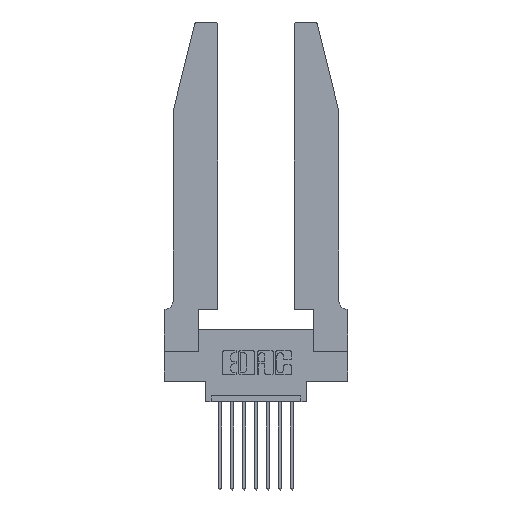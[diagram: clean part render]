
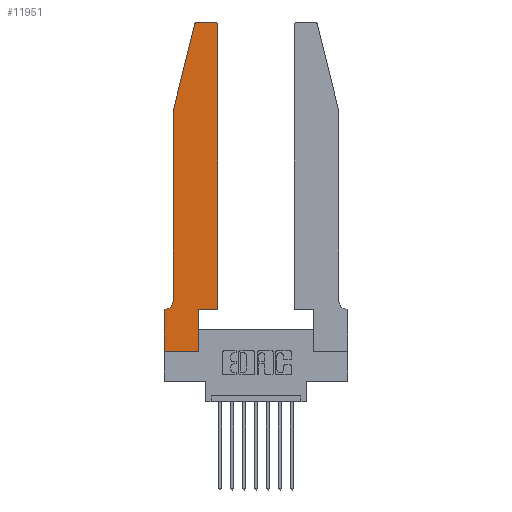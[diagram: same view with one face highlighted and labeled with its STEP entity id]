
A CAD part, top view. The second image highlights one B-rep face of the part: STEP entity #11951.
In plain terms, the highlighted planar face has unit normal (0, 0, 1).
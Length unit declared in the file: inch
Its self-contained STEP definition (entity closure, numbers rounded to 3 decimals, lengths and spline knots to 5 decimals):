
#201 = ORIENTED_EDGE ( 'NONE', *, *, #12708, .T. ) ;
#231 = CARTESIAN_POINT ( 'NONE',  ( 0.2865, 0.35, 0.37 ) ) ;
#441 = VECTOR ( 'NONE', #7008, 39.37008 ) ;
#580 = VECTOR ( 'NONE', #14344, 39.37008 ) ;
#858 = EDGE_CURVE ( 'NONE', #9339, #12194, #10511, .T. ) ;
#965 = EDGE_CURVE ( 'NONE', #3854, #10141, #13375, .T. ) ;
#1080 = CARTESIAN_POINT ( 'NONE',  ( 0.0755, 2., 0.37 ) ) ;
#1188 = FACE_OUTER_BOUND ( 'NONE', #7702, .T. ) ;
#1193 = DIRECTION ( 'NONE',  ( 0., -1., 0. ) ) ;
#1369 = CARTESIAN_POINT ( 'NONE',  ( 0., 0.35, 0.37 ) ) ;
#1457 = VERTEX_POINT ( 'NONE', #10189 ) ;
#1799 = ORIENTED_EDGE ( 'NONE', *, *, #965, .T. ) ;
#1825 = ORIENTED_EDGE ( 'NONE', *, *, #12223, .T. ) ;
#1881 = VECTOR ( 'NONE', #5202, 39.37008 ) ;
#2088 = CIRCLE ( 'NONE', #11531, 0.07 ) ;
#2167 = ORIENTED_EDGE ( 'NONE', *, *, #7016, .T. ) ;
#2403 = EDGE_CURVE ( 'NONE', #10127, #9339, #9746, .T. ) ;
#2482 = CARTESIAN_POINT ( 'NONE',  ( 0., 0., 0.37 ) ) ;
#2566 = LINE ( 'NONE', #8594, #6352 ) ;
#2736 = ORIENTED_EDGE ( 'NONE', *, *, #8646, .T. ) ;
#2794 = LINE ( 'NONE', #10407, #14669 ) ;
#2820 = CARTESIAN_POINT ( 'NONE',  ( 0., 0., 0.37 ) ) ;
#2854 = DIRECTION ( 'NONE',  ( 0., 0., 1. ) ) ;
#2910 = CARTESIAN_POINT ( 'NONE',  ( 0.2865, 0.35, 0.37 ) ) ;
#3718 = ORIENTED_EDGE ( 'NONE', *, *, #12362, .T. ) ;
#3731 = VERTEX_POINT ( 'NONE', #9314 ) ;
#3753 = CARTESIAN_POINT ( 'NONE',  ( 0.0055, 0.35, 0.37 ) ) ;
#3854 = VERTEX_POINT ( 'NONE', #10571 ) ;
#4347 = DIRECTION ( 'NONE',  ( -1., 0., 0. ) ) ;
#4567 = VECTOR ( 'NONE', #5800, 39.37008 ) ;
#4826 = ORIENTED_EDGE ( 'NONE', *, *, #14620, .T. ) ;
#4857 = EDGE_CURVE ( 'NONE', #14007, #7951, #13244, .T. ) ;
#4919 = LINE ( 'NONE', #6512, #1881 ) ;
#4931 = CARTESIAN_POINT ( 'NONE',  ( 0.25487, 2.72718, 0.37 ) ) ;
#5147 = CARTESIAN_POINT ( 'NONE',  ( 0.0755, 2., 0.37 ) ) ;
#5202 = DIRECTION ( 'NONE',  ( -1., 0., 0. ) ) ;
#5597 = LINE ( 'NONE', #7688, #5964 ) ;
#5800 = DIRECTION ( 'NONE',  ( -0.239, -0.971, 0. ) ) ;
#5964 = VECTOR ( 'NONE', #4347, 39.37008 ) ;
#6033 = EDGE_CURVE ( 'NONE', #3731, #8419, #2088, .T. ) ;
#6352 = VECTOR ( 'NONE', #14443, 39.37008 ) ;
#6512 = CARTESIAN_POINT ( 'NONE',  ( 0.0755, 0.35, 0.37 ) ) ;
#6681 = DIRECTION ( 'NONE',  ( 1., 0., 0. ) ) ;
#7008 = DIRECTION ( 'NONE',  ( 0., 1., 0. ) ) ;
#7016 = EDGE_CURVE ( 'NONE', #12194, #3854, #2566, .T. ) ;
#7195 = CARTESIAN_POINT ( 'NONE',  ( 0.4505, 2.72, 0.37 ) ) ;
#7467 = VECTOR ( 'NONE', #14351, 39.37008 ) ;
#7688 = CARTESIAN_POINT ( 'NONE',  ( 0.2605, 2.75, 0.37 ) ) ;
#7702 = EDGE_LOOP ( 'NONE', ( #2736, #10166, #201, #11525, #13347, #4826, #3718, #14055, #12263, #2167, #1799, #1825 ) ) ;
#7819 = CARTESIAN_POINT ( 'NONE',  ( 0.4205, 2.75, 0.37 ) ) ;
#7951 = VERTEX_POINT ( 'NONE', #4931 ) ;
#8194 = PLANE ( 'NONE',  #14264 ) ;
#8221 = AXIS2_PLACEMENT_3D ( 'NONE', #13049, #2854, #14331 ) ;
#8419 = VERTEX_POINT ( 'NONE', #3753 ) ;
#8424 = DIRECTION ( 'NONE',  ( 1., 0., 0. ) ) ;
#8594 = CARTESIAN_POINT ( 'NONE',  ( 0.4505, 0.35, 0.37 ) ) ;
#8646 = EDGE_CURVE ( 'NONE', #14082, #14007, #5597, .T. ) ;
#8884 = DIRECTION ( 'NONE',  ( -1., 0., 0. ) ) ;
#9314 = CARTESIAN_POINT ( 'NONE',  ( 0.0755, 0.42, 0.37 ) ) ;
#9339 = VERTEX_POINT ( 'NONE', #11281 ) ;
#9552 = VERTEX_POINT ( 'NONE', #14471 ) ;
#9625 = DIRECTION ( 'NONE',  ( 0., 1., 0. ) ) ;
#9636 = CIRCLE ( 'NONE', #12228, 0.03 ) ;
#9746 = LINE ( 'NONE', #2820, #580 ) ;
#9859 = DIRECTION ( 'NONE',  ( 0., 0., -1. ) ) ;
#10127 = VERTEX_POINT ( 'NONE', #2482 ) ;
#10141 = VERTEX_POINT ( 'NONE', #7195 ) ;
#10166 = ORIENTED_EDGE ( 'NONE', *, *, #4857, .T. ) ;
#10189 = CARTESIAN_POINT ( 'NONE',  ( 0., 0.35, 0.37 ) ) ;
#10210 = DIRECTION ( 'NONE',  ( 0., 0., 1. ) ) ;
#10407 = CARTESIAN_POINT ( 'NONE',  ( 0., 0., 0.37 ) ) ;
#10511 = LINE ( 'NONE', #231, #441 ) ;
#10571 = CARTESIAN_POINT ( 'NONE',  ( 0.4505, 0.35, 0.37 ) ) ;
#11068 = CARTESIAN_POINT ( 'NONE',  ( 0.0055, 0.42, 0.37 ) ) ;
#11281 = CARTESIAN_POINT ( 'NONE',  ( 0.2865, 0., 0.37 ) ) ;
#11525 = ORIENTED_EDGE ( 'NONE', *, *, #12986, .T. ) ;
#11531 = AXIS2_PLACEMENT_3D ( 'NONE', #11068, #9859, #8884 ) ;
#11946 = VECTOR ( 'NONE', #9625, 39.37008 ) ;
#11951 = ADVANCED_FACE ( 'NONE', ( #1188 ), #8194, .T. ) ;
#12121 = LINE ( 'NONE', #5147, #7467 ) ;
#12134 = LINE ( 'NONE', #1080, #4567 ) ;
#12194 = VERTEX_POINT ( 'NONE', #2910 ) ;
#12223 = EDGE_CURVE ( 'NONE', #10141, #14082, #9636, .T. ) ;
#12228 = AXIS2_PLACEMENT_3D ( 'NONE', #13660, #10210, #6681 ) ;
#12263 = ORIENTED_EDGE ( 'NONE', *, *, #858, .T. ) ;
#12362 = EDGE_CURVE ( 'NONE', #1457, #10127, #2794, .T. ) ;
#12708 = EDGE_CURVE ( 'NONE', #7951, #9552, #12134, .T. ) ;
#12986 = EDGE_CURVE ( 'NONE', #9552, #3731, #12121, .T. ) ;
#13049 = CARTESIAN_POINT ( 'NONE',  ( 0.284, 2.72, 0.37 ) ) ;
#13156 = DIRECTION ( 'NONE',  ( 0., 0., 1. ) ) ;
#13244 = CIRCLE ( 'NONE', #8221, 0.03 ) ;
#13347 = ORIENTED_EDGE ( 'NONE', *, *, #6033, .T. ) ;
#13375 = LINE ( 'NONE', #14347, #11946 ) ;
#13660 = CARTESIAN_POINT ( 'NONE',  ( 0.4205, 2.72, 0.37 ) ) ;
#14007 = VERTEX_POINT ( 'NONE', #14617 ) ;
#14055 = ORIENTED_EDGE ( 'NONE', *, *, #2403, .T. ) ;
#14082 = VERTEX_POINT ( 'NONE', #7819 ) ;
#14264 = AXIS2_PLACEMENT_3D ( 'NONE', #1369, #13156, #8424 ) ;
#14331 = DIRECTION ( 'NONE',  ( 1., 0., 0. ) ) ;
#14344 = DIRECTION ( 'NONE',  ( 1., 0., 0. ) ) ;
#14347 = CARTESIAN_POINT ( 'NONE',  ( 0.4505, 0.35, 0.37 ) ) ;
#14351 = DIRECTION ( 'NONE',  ( 0., -1., 0. ) ) ;
#14443 = DIRECTION ( 'NONE',  ( 1., 0., 0. ) ) ;
#14471 = CARTESIAN_POINT ( 'NONE',  ( 0.0755, 2., 0.37 ) ) ;
#14617 = CARTESIAN_POINT ( 'NONE',  ( 0.284, 2.75, 0.37 ) ) ;
#14620 = EDGE_CURVE ( 'NONE', #8419, #1457, #4919, .T. ) ;
#14669 = VECTOR ( 'NONE', #1193, 39.37008 ) ;
